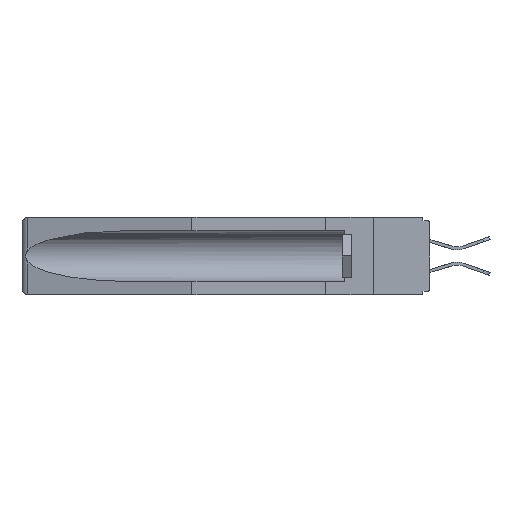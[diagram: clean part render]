
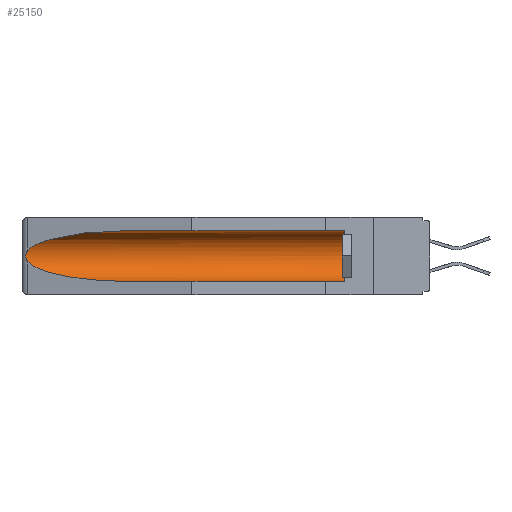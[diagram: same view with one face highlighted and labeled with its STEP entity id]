
A CAD part, left-side view. The second image highlights one B-rep face of the part: STEP entity #25150.
In plain terms, the highlighted cylindrical face has radius 2.857 mm (diameter 5.715 mm), a partial arc.
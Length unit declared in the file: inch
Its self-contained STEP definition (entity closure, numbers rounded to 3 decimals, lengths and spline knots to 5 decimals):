
#352 = ORIENTED_EDGE ( 'NONE', *, *, #2801, .T. ) ;
#1607 = CARTESIAN_POINT ( 'NONE',  ( 0.26654, 1.53092, -0.15636 ) ) ;
#1694 = CARTESIAN_POINT ( 'NONE',  ( 0.26597, 1.5296, -0.19026 ) ) ;
#2445 =( BOUNDED_CURVE ( )  B_SPLINE_CURVE ( 3, ( #4032, #6491, #28136, #21597 ),
 .UNSPECIFIED., .F., .F. ) 
 B_SPLINE_CURVE_WITH_KNOTS ( ( 4, 4 ),
 ( 4.71239, 6.08839 ),
 .UNSPECIFIED. ) 
 CURVE ( )  GEOMETRIC_REPRESENTATION_ITEM ( )  RATIONAL_B_SPLINE_CURVE ( ( 1., 0.848, 0.848, 1. ) ) 
 REPRESENTATION_ITEM ( '' )  );
#2606 = CARTESIAN_POINT ( 'NONE',  ( 0.21114, 1.30732, -0.284 ) ) ;
#2801 = EDGE_CURVE ( 'NONE', #8232, #19452, #9035, .T. ) ;
#4032 = CARTESIAN_POINT ( 'NONE',  ( 0.155, 1.07973, -0.059 ) ) ;
#4158 = CYLINDRICAL_SURFACE ( 'NONE', #27321, 0.1125 ) ;
#4563 = CARTESIAN_POINT ( 'NONE',  ( 0.26537, 1.52718, -0.14972 ) ) ;
#5039 = EDGE_CURVE ( 'NONE', #15097, #16719, #12621, .T. ) ;
#6170 = DIRECTION ( 'NONE',  ( 0., 0., 1. ) ) ;
#6491 = CARTESIAN_POINT ( 'NONE',  ( 0.21114, 1.30732, -0.059 ) ) ;
#6624 = VERTEX_POINT ( 'NONE', #15486 ) ;
#7519 = CARTESIAN_POINT ( 'NONE',  ( 0.26537, 1.52718, -0.19328 ) ) ;
#7765 = DIRECTION ( 'NONE',  ( 0., 1., 0. ) ) ;
#7867 = CARTESIAN_POINT ( 'NONE',  ( 0.155, -0.30754, -0.059 ) ) ;
#8232 = VERTEX_POINT ( 'NONE', #21573 ) ;
#9035 = CIRCLE ( 'NONE', #14110, 0.1125 ) ;
#12252 = LINE ( 'NONE', #12522, #22838 ) ;
#12270 = ORIENTED_EDGE ( 'NONE', *, *, #19622, .T. ) ;
#12433 = CARTESIAN_POINT ( 'NONE',  ( 0.2673, 1.5327, -0.16383 ) ) ;
#12522 = CARTESIAN_POINT ( 'NONE',  ( 0.155, -0.30754, -0.284 ) ) ;
#12588 = ORIENTED_EDGE ( 'NONE', *, *, #13087, .T. ) ;
#12621 = B_SPLINE_CURVE_WITH_KNOTS ( 'NONE', 3,
 ( #16995, #21085, #1607, #12433, #14603, #23400, #14792, #14508, #1694, #25443 ),
 .UNSPECIFIED., .F., .F.,
 ( 4, 2, 2, 2, 4 ),
 ( 0., 0.00029, 0.00058, 0.00087, 0.00117 ),
 .UNSPECIFIED. ) ;
#12641 = CARTESIAN_POINT ( 'NONE',  ( 0.155, 1.07973, -0.284 ) ) ;
#13087 = EDGE_CURVE ( 'NONE', #16719, #13568, #25055, .T. ) ;
#13568 = VERTEX_POINT ( 'NONE', #12641 ) ;
#14011 = EDGE_CURVE ( 'NONE', #6624, #15097, #2445, .T. ) ;
#14110 = AXIS2_PLACEMENT_3D ( 'NONE', #27987, #14685, #6170 ) ;
#14508 = CARTESIAN_POINT ( 'NONE',  ( 0.26655, 1.53094, -0.18657 ) ) ;
#14603 = CARTESIAN_POINT ( 'NONE',  ( 0.2675, 1.53308, -0.16763 ) ) ;
#14685 = DIRECTION ( 'NONE',  ( 0., -1., 0. ) ) ;
#14792 = CARTESIAN_POINT ( 'NONE',  ( 0.2673, 1.53269, -0.17917 ) ) ;
#15097 = VERTEX_POINT ( 'NONE', #4563 ) ;
#15486 = CARTESIAN_POINT ( 'NONE',  ( 0.155, 1.07973, -0.059 ) ) ;
#15712 = CARTESIAN_POINT ( 'NONE',  ( 0.25451, 1.48313, -0.24835 ) ) ;
#16719 = VERTEX_POINT ( 'NONE', #7519 ) ;
#16797 = FACE_OUTER_BOUND ( 'NONE', #22607, .T. ) ;
#16995 = CARTESIAN_POINT ( 'NONE',  ( 0.26537, 1.52718, -0.14972 ) ) ;
#17897 = CARTESIAN_POINT ( 'NONE',  ( 0.155, 1.07973, -0.284 ) ) ;
#18720 = ORIENTED_EDGE ( 'NONE', *, *, #20466, .F. ) ;
#19361 = CARTESIAN_POINT ( 'NONE',  ( 0.155, -0.30754, -0.1715 ) ) ;
#19452 = VERTEX_POINT ( 'NONE', #23726 ) ;
#19622 = EDGE_CURVE ( 'NONE', #19452, #6624, #24655, .T. ) ;
#20266 = ORIENTED_EDGE ( 'NONE', *, *, #14011, .T. ) ;
#20466 = EDGE_CURVE ( 'NONE', #8232, #13568, #12252, .T. ) ;
#20472 = VECTOR ( 'NONE', #7765, 39.37008 ) ;
#21085 = CARTESIAN_POINT ( 'NONE',  ( 0.26597, 1.52961, -0.15275 ) ) ;
#21573 = CARTESIAN_POINT ( 'NONE',  ( 0.155, 0.126, -0.284 ) ) ;
#21597 = CARTESIAN_POINT ( 'NONE',  ( 0.26537, 1.52718, -0.14972 ) ) ;
#21775 = DIRECTION ( 'NONE',  ( 0., 1., 0. ) ) ;
#22327 = ORIENTED_EDGE ( 'NONE', *, *, #5039, .T. ) ;
#22607 = EDGE_LOOP ( 'NONE', ( #20266, #22327, #12588, #18720, #352, #12270 ) ) ;
#22838 = VECTOR ( 'NONE', #27805, 39.37008 ) ;
#23400 = CARTESIAN_POINT ( 'NONE',  ( 0.2675, 1.53308, -0.17534 ) ) ;
#23726 = CARTESIAN_POINT ( 'NONE',  ( 0.155, 0.126, -0.059 ) ) ;
#24655 = LINE ( 'NONE', #7867, #20472 ) ;
#25055 =( BOUNDED_CURVE ( )  B_SPLINE_CURVE ( 3, ( #26858, #15712, #2606, #17897 ),
 .UNSPECIFIED., .F., .F. ) 
 B_SPLINE_CURVE_WITH_KNOTS ( ( 4, 4 ),
 ( 0.1948, 1.5708 ),
 .UNSPECIFIED. ) 
 CURVE ( )  GEOMETRIC_REPRESENTATION_ITEM ( )  RATIONAL_B_SPLINE_CURVE ( ( 1., 0.848, 0.848, 1. ) ) 
 REPRESENTATION_ITEM ( '' )  );
#25150 = ADVANCED_FACE ( 'NONE', ( #16797 ), #4158, .F. ) ;
#25443 = CARTESIAN_POINT ( 'NONE',  ( 0.26537, 1.52718, -0.19328 ) ) ;
#26147 = DIRECTION ( 'NONE',  ( 0., 0., 1. ) ) ;
#26858 = CARTESIAN_POINT ( 'NONE',  ( 0.26537, 1.52718, -0.19328 ) ) ;
#27321 = AXIS2_PLACEMENT_3D ( 'NONE', #19361, #21775, #26147 ) ;
#27805 = DIRECTION ( 'NONE',  ( 0., 1., 0. ) ) ;
#27987 = CARTESIAN_POINT ( 'NONE',  ( 0.155, 0.126, -0.1715 ) ) ;
#28136 = CARTESIAN_POINT ( 'NONE',  ( 0.25451, 1.48313, -0.09465 ) ) ;
